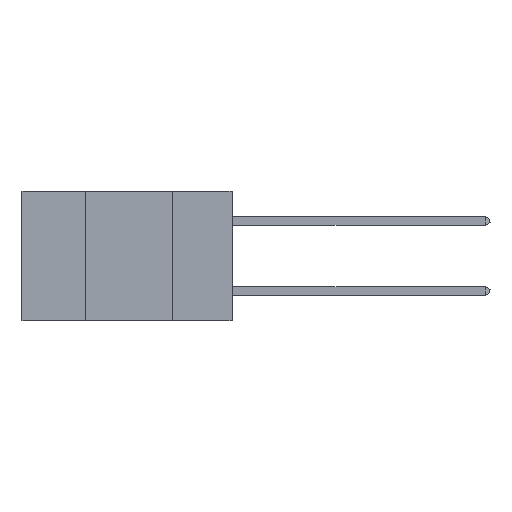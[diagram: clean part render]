
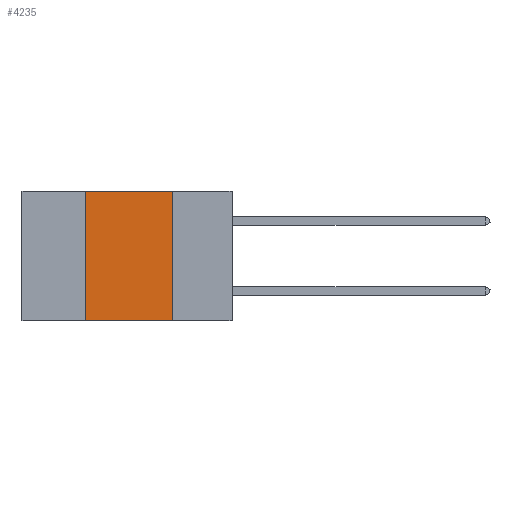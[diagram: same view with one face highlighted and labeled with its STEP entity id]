
A CAD part, left-side view. The second image highlights one B-rep face of the part: STEP entity #4235.
In plain terms, the highlighted planar face has unit normal (-1, 0, 0).
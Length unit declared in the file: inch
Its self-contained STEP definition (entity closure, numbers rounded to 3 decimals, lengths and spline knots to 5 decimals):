
#429 = CARTESIAN_POINT ( 'NONE',  ( 0., 0.17, 0. ) ) ;
#1549 = LINE ( 'NONE', #14712, #10438 ) ;
#1636 = CARTESIAN_POINT ( 'NONE',  ( 0., 0.6, -0.37 ) ) ;
#1642 = CARTESIAN_POINT ( 'NONE',  ( 0., 0.6, 0. ) ) ;
#1710 = DIRECTION ( 'NONE',  ( 0., -1., 0. ) ) ;
#2880 = VECTOR ( 'NONE', #15888, 39.37008 ) ;
#3080 = CARTESIAN_POINT ( 'NONE',  ( 0., 0.42, -0.37 ) ) ;
#3294 = EDGE_CURVE ( 'NONE', #8099, #17532, #6900, .T. ) ;
#4235 = ADVANCED_FACE ( 'NONE', ( #7178 ), #17445, .F. ) ;
#4276 = EDGE_CURVE ( 'NONE', #8099, #15114, #1549, .T. ) ;
#4812 = EDGE_CURVE ( 'NONE', #15114, #9337, #5004, .T. ) ;
#4910 = EDGE_LOOP ( 'NONE', ( #19660, #10701, #18736, #7961 ) ) ;
#5004 = LINE ( 'NONE', #1642, #13039 ) ;
#6464 = AXIS2_PLACEMENT_3D ( 'NONE', #18975, #17407, #15863 ) ;
#6900 = LINE ( 'NONE', #1636, #2880 ) ;
#7178 = FACE_OUTER_BOUND ( 'NONE', #4910, .T. ) ;
#7961 = ORIENTED_EDGE ( 'NONE', *, *, #3294, .T. ) ;
#8099 = VERTEX_POINT ( 'NONE', #3080 ) ;
#9337 = VERTEX_POINT ( 'NONE', #429 ) ;
#10438 = VECTOR ( 'NONE', #15256, 39.37008 ) ;
#10701 = ORIENTED_EDGE ( 'NONE', *, *, #4812, .F. ) ;
#11944 = LINE ( 'NONE', #16732, #20387 ) ;
#13039 = VECTOR ( 'NONE', #1710, 39.37008 ) ;
#14712 = CARTESIAN_POINT ( 'NONE',  ( 0., 0.42, 0. ) ) ;
#14736 = CARTESIAN_POINT ( 'NONE',  ( 0., 0.17, -0.37 ) ) ;
#15114 = VERTEX_POINT ( 'NONE', #18795 ) ;
#15256 = DIRECTION ( 'NONE',  ( 0., 0., 1. ) ) ;
#15863 = DIRECTION ( 'NONE',  ( 0., 0., -1. ) ) ;
#15888 = DIRECTION ( 'NONE',  ( 0., -1., 0. ) ) ;
#16732 = CARTESIAN_POINT ( 'NONE',  ( 0., 0.17, 0. ) ) ;
#17407 = DIRECTION ( 'NONE',  ( 1., 0., 0. ) ) ;
#17445 = PLANE ( 'NONE',  #6464 ) ;
#17532 = VERTEX_POINT ( 'NONE', #14736 ) ;
#18177 = DIRECTION ( 'NONE',  ( 0., 0., -1. ) ) ;
#18736 = ORIENTED_EDGE ( 'NONE', *, *, #4276, .F. ) ;
#18795 = CARTESIAN_POINT ( 'NONE',  ( 0., 0.42, 0. ) ) ;
#18975 = CARTESIAN_POINT ( 'NONE',  ( 0., 0.6, 0. ) ) ;
#19660 = ORIENTED_EDGE ( 'NONE', *, *, #20198, .F. ) ;
#20198 = EDGE_CURVE ( 'NONE', #9337, #17532, #11944, .T. ) ;
#20387 = VECTOR ( 'NONE', #18177, 39.37008 ) ;
